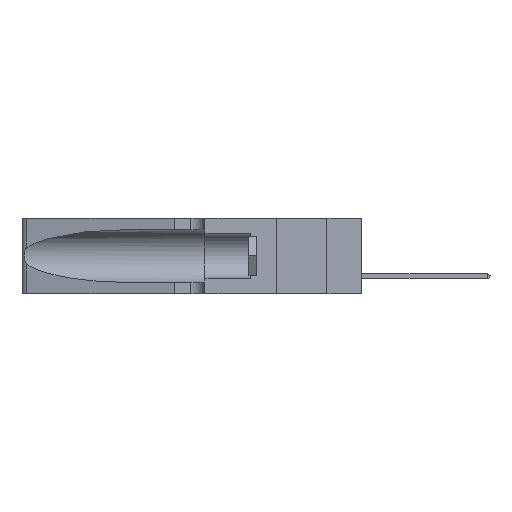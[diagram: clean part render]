
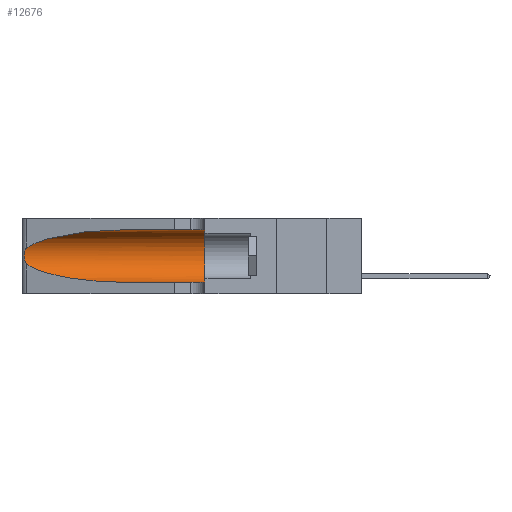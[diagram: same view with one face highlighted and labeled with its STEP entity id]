
A CAD part, left-side view. The second image highlights one B-rep face of the part: STEP entity #12676.
In plain terms, the highlighted cylindrical face has radius 3.308 mm (diameter 6.617 mm), a partial arc.
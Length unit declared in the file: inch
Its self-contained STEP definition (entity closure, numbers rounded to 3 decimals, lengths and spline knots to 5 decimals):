
#1315 = EDGE_CURVE ( 'NONE', #46618, #5448, #19571, .T. ) ;
#3786 = DIRECTION ( 'NONE',  ( 0., 0., 1. ) ) ;
#5022 = DIRECTION ( 'NONE',  ( 0., -1., 0. ) ) ;
#5448 = VERTEX_POINT ( 'NONE', #36606 ) ;
#6134 = CARTESIAN_POINT ( 'NONE',  ( 0.25487, 1.22718, 0.14631 ) ) ;
#8080 = CARTESIAN_POINT ( 'NONE',  ( 0.1305, 0.35, 0.31525 ) ) ;
#9344 = CARTESIAN_POINT ( 'NONE',  ( 0.1305, 0.72297, 0.31525 ) ) ;
#10076 = DIRECTION ( 'NONE',  ( 0., -1., 0. ) ) ;
#10333 = CARTESIAN_POINT ( 'NONE',  ( 0.25854, 1.2359, 0.20912 ) ) ;
#10472 = EDGE_LOOP ( 'NONE', ( #36526, #31934, #29388, #40831, #36216, #24740 ) ) ;
#10484 = EDGE_CURVE ( 'NONE', #18151, #15267, #40130, .T. ) ;
#12676 = ADVANCED_FACE ( 'NONE', ( #13523 ), #25682, .F. ) ;
#13523 = FACE_OUTER_BOUND ( 'NONE', #10472, .T. ) ;
#13804 = CARTESIAN_POINT ( 'NONE',  ( 0.1305, 0.72297, 0.05475 ) ) ;
#13977 = CARTESIAN_POINT ( 'NONE',  ( 0.25487, 1.22718, 0.22369 ) ) ;
#14229 = CARTESIAN_POINT ( 'NONE',  ( 0.26018, 1.23835, 0.19895 ) ) ;
#14597 = CARTESIAN_POINT ( 'NONE',  ( 0.1305, 0.35, 0.05475 ) ) ;
#15267 = VERTEX_POINT ( 'NONE', #8080 ) ;
#16044 =( BOUNDED_CURVE ( )  B_SPLINE_CURVE ( 3, ( #49423, #33744, #22260, #37786 ),
 .UNSPECIFIED., .F., .T. ) 
 B_SPLINE_CURVE_WITH_KNOTS ( ( 4, 4 ),
 ( 3.44316, 4.71239 ),
 .UNSPECIFIED. ) 
 CURVE ( )  GEOMETRIC_REPRESENTATION_ITEM ( )  RATIONAL_B_SPLINE_CURVE ( ( 1., 0.87, 0.87, 1. ) ) 
 REPRESENTATION_ITEM ( '' )  );
#16962 = CARTESIAN_POINT ( 'NONE',  ( 0.18966, 0.96281, 0.31525 ) ) ;
#17934 = CARTESIAN_POINT ( 'NONE',  ( 0.26075, 1.23896, 0.19203 ) ) ;
#18151 = VERTEX_POINT ( 'NONE', #28824 ) ;
#18289 = CARTESIAN_POINT ( 'NONE',  ( 0.25787, 1.23484, 0.2124 ) ) ;
#18646 = EDGE_CURVE ( 'NONE', #18151, #46618, #37168, .T. ) ;
#19189 = CARTESIAN_POINT ( 'NONE',  ( 0.1305, 0.35, 0.185 ) ) ;
#19571 = B_SPLINE_CURVE_WITH_KNOTS ( 'NONE', 3,
 ( #22163, #26223, #45450, #18289, #10333, #14229, #17934, #22004, #45294, #49169, #29932, #21676, #29760, #6134 ),
 .UNSPECIFIED., .F., .F.,
 ( 4, 2, 2, 2, 2, 2, 4 ),
 ( 0., 0.00027, 0.00053, 0.00107, 0.0016, 0.00187, 0.00214 ),
 .UNSPECIFIED. ) ;
#20883 = CARTESIAN_POINT ( 'NONE',  ( 0.2373, 1.15595, 0.28018 ) ) ;
#21291 = EDGE_CURVE ( 'NONE', #15267, #39331, #23773, .T. ) ;
#21676 = CARTESIAN_POINT ( 'NONE',  ( 0.25639, 1.23186, 0.15144 ) ) ;
#22004 = CARTESIAN_POINT ( 'NONE',  ( 0.26075, 1.23896, 0.178 ) ) ;
#22163 = CARTESIAN_POINT ( 'NONE',  ( 0.25487, 1.22718, 0.22369 ) ) ;
#22260 = CARTESIAN_POINT ( 'NONE',  ( 0.18966, 0.96281, 0.05475 ) ) ;
#23773 = CIRCLE ( 'NONE', #47248, 0.13025 ) ;
#24448 = DIRECTION ( 'NONE',  ( 0., 0., -1. ) ) ;
#24740 = ORIENTED_EDGE ( 'NONE', *, *, #10484, .F. ) ;
#25619 = CARTESIAN_POINT ( 'NONE',  ( 0.1305, 1.61858, 0.05475 ) ) ;
#25682 = CYLINDRICAL_SURFACE ( 'NONE', #29934, 0.13025 ) ;
#26223 = CARTESIAN_POINT ( 'NONE',  ( 0.25555, 1.22994, 0.2215 ) ) ;
#27462 = EDGE_CURVE ( 'NONE', #5448, #48535, #16044, .T. ) ;
#28248 = VECTOR ( 'NONE', #10076, 39.37008 ) ;
#28644 = VECTOR ( 'NONE', #33141, 39.37008 ) ;
#28824 = CARTESIAN_POINT ( 'NONE',  ( 0.1305, 0.72297, 0.31525 ) ) ;
#29388 = ORIENTED_EDGE ( 'NONE', *, *, #27462, .T. ) ;
#29760 = CARTESIAN_POINT ( 'NONE',  ( 0.25555, 1.22993, 0.14849 ) ) ;
#29932 = CARTESIAN_POINT ( 'NONE',  ( 0.25789, 1.23486, 0.15765 ) ) ;
#29934 = AXIS2_PLACEMENT_3D ( 'NONE', #35801, #5022, #24448 ) ;
#31934 = ORIENTED_EDGE ( 'NONE', *, *, #1315, .T. ) ;
#32502 = CARTESIAN_POINT ( 'NONE',  ( 0.25487, 1.22718, 0.22369 ) ) ;
#32952 = CARTESIAN_POINT ( 'NONE',  ( 0.1305, 1.61858, 0.31525 ) ) ;
#33141 = DIRECTION ( 'NONE',  ( 0., -1., 0. ) ) ;
#33744 = CARTESIAN_POINT ( 'NONE',  ( 0.2373, 1.15595, 0.08982 ) ) ;
#35801 = CARTESIAN_POINT ( 'NONE',  ( 0.1305, 1.61858, 0.185 ) ) ;
#36216 = ORIENTED_EDGE ( 'NONE', *, *, #21291, .F. ) ;
#36526 = ORIENTED_EDGE ( 'NONE', *, *, #18646, .T. ) ;
#36606 = CARTESIAN_POINT ( 'NONE',  ( 0.25487, 1.22718, 0.14631 ) ) ;
#37168 =( BOUNDED_CURVE ( )  B_SPLINE_CURVE ( 3, ( #9344, #16962, #20883, #32502 ),
 .UNSPECIFIED., .F., .T. ) 
 B_SPLINE_CURVE_WITH_KNOTS ( ( 4, 4 ),
 ( 1.5708, 2.84003 ),
 .UNSPECIFIED. ) 
 CURVE ( )  GEOMETRIC_REPRESENTATION_ITEM ( )  RATIONAL_B_SPLINE_CURVE ( ( 1., 0.87, 0.87, 1. ) ) 
 REPRESENTATION_ITEM ( '' )  );
#37786 = CARTESIAN_POINT ( 'NONE',  ( 0.1305, 0.72297, 0.05475 ) ) ;
#39331 = VERTEX_POINT ( 'NONE', #14597 ) ;
#40130 = LINE ( 'NONE', #32952, #28644 ) ;
#40831 = ORIENTED_EDGE ( 'NONE', *, *, #46615, .T. ) ;
#44610 = LINE ( 'NONE', #25619, #28248 ) ;
#45294 = CARTESIAN_POINT ( 'NONE',  ( 0.26017, 1.23833, 0.17102 ) ) ;
#45450 = CARTESIAN_POINT ( 'NONE',  ( 0.25639, 1.23184, 0.21858 ) ) ;
#46194 = DIRECTION ( 'NONE',  ( 0., 1., 0. ) ) ;
#46615 = EDGE_CURVE ( 'NONE', #48535, #39331, #44610, .T. ) ;
#46618 = VERTEX_POINT ( 'NONE', #13977 ) ;
#47248 = AXIS2_PLACEMENT_3D ( 'NONE', #19189, #46194, #3786 ) ;
#48535 = VERTEX_POINT ( 'NONE', #13804 ) ;
#49169 = CARTESIAN_POINT ( 'NONE',  ( 0.25856, 1.23593, 0.16098 ) ) ;
#49423 = CARTESIAN_POINT ( 'NONE',  ( 0.25487, 1.22718, 0.14631 ) ) ;
